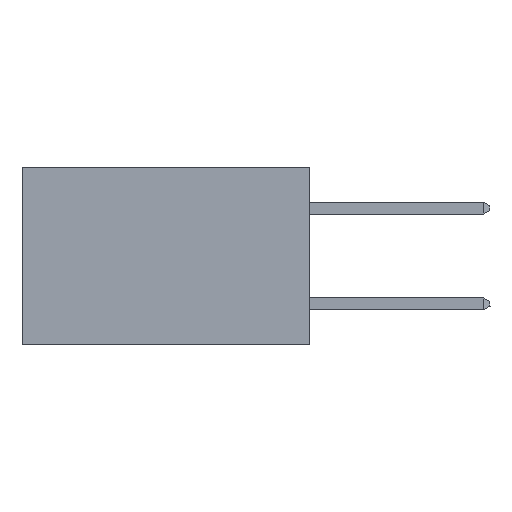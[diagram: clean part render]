
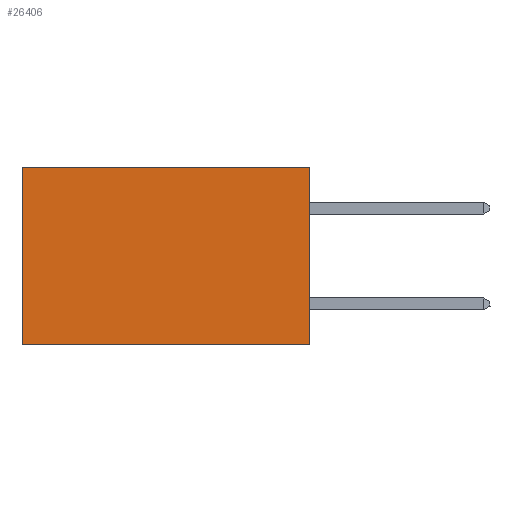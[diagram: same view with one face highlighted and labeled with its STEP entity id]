
A CAD part, left-side view. The second image highlights one B-rep face of the part: STEP entity #26406.
In plain terms, the highlighted planar face has unit normal (-1, 0, 0).
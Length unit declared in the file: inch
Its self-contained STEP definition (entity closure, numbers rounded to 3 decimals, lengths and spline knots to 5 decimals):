
#2389 = LINE ( 'NONE', #23727, #30027 ) ;
#3988 = DIRECTION ( 'NONE',  ( 1., 0., 0. ) ) ;
#4903 = ORIENTED_EDGE ( 'NONE', *, *, #8861, .T. ) ;
#5165 = DIRECTION ( 'NONE',  ( 0., 0., -1. ) ) ;
#6536 = VECTOR ( 'NONE', #12636, 39.37008 ) ;
#7530 = DIRECTION ( 'NONE',  ( 0., 1., 0. ) ) ;
#8565 = EDGE_CURVE ( 'NONE', #34530, #29081, #31694, .T. ) ;
#8861 = EDGE_CURVE ( 'NONE', #34530, #10461, #2389, .T. ) ;
#10051 = CARTESIAN_POINT ( 'NONE',  ( 0.2875, 0., 0. ) ) ;
#10461 = VERTEX_POINT ( 'NONE', #17761 ) ;
#11855 = CARTESIAN_POINT ( 'NONE',  ( 0.2875, 0., -0.37 ) ) ;
#12636 = DIRECTION ( 'NONE',  ( 0., 0., -1. ) ) ;
#13499 = CARTESIAN_POINT ( 'NONE',  ( 0.2875, 0.6, 0. ) ) ;
#14531 = DIRECTION ( 'NONE',  ( 0., 0., -1. ) ) ;
#17761 = CARTESIAN_POINT ( 'NONE',  ( 0.2875, 0.6, 0. ) ) ;
#22723 = LINE ( 'NONE', #31940, #32335 ) ;
#22917 = ORIENTED_EDGE ( 'NONE', *, *, #24554, .F. ) ;
#23727 = CARTESIAN_POINT ( 'NONE',  ( 0.2875, 0., 0. ) ) ;
#24554 = EDGE_CURVE ( 'NONE', #29081, #29704, #22723, .T. ) ;
#25157 = LINE ( 'NONE', #13499, #34315 ) ;
#25793 = ORIENTED_EDGE ( 'NONE', *, *, #34109, .T. ) ;
#26406 = ADVANCED_FACE ( 'NONE', ( #27205 ), #33468, .F. ) ;
#26583 = ORIENTED_EDGE ( 'NONE', *, *, #8565, .F. ) ;
#27205 = FACE_OUTER_BOUND ( 'NONE', #33408, .T. ) ;
#28413 = CARTESIAN_POINT ( 'NONE',  ( 0.2875, 0.6, -0.37 ) ) ;
#28486 = CARTESIAN_POINT ( 'NONE',  ( 0.2875, 0., 0. ) ) ;
#28953 = DIRECTION ( 'NONE',  ( 0., 1., 0. ) ) ;
#29081 = VERTEX_POINT ( 'NONE', #11855 ) ;
#29704 = VERTEX_POINT ( 'NONE', #28413 ) ;
#30027 = VECTOR ( 'NONE', #7530, 39.37008 ) ;
#31694 = LINE ( 'NONE', #10051, #6536 ) ;
#31940 = CARTESIAN_POINT ( 'NONE',  ( 0.2875, 0., -0.37 ) ) ;
#32335 = VECTOR ( 'NONE', #28953, 39.37008 ) ;
#33346 = CARTESIAN_POINT ( 'NONE',  ( 0.2875, 0., 0. ) ) ;
#33408 = EDGE_LOOP ( 'NONE', ( #25793, #22917, #26583, #4903 ) ) ;
#33468 = PLANE ( 'NONE',  #34292 ) ;
#34109 = EDGE_CURVE ( 'NONE', #10461, #29704, #25157, .T. ) ;
#34292 = AXIS2_PLACEMENT_3D ( 'NONE', #33346, #3988, #14531 ) ;
#34315 = VECTOR ( 'NONE', #5165, 39.37008 ) ;
#34530 = VERTEX_POINT ( 'NONE', #28486 ) ;
